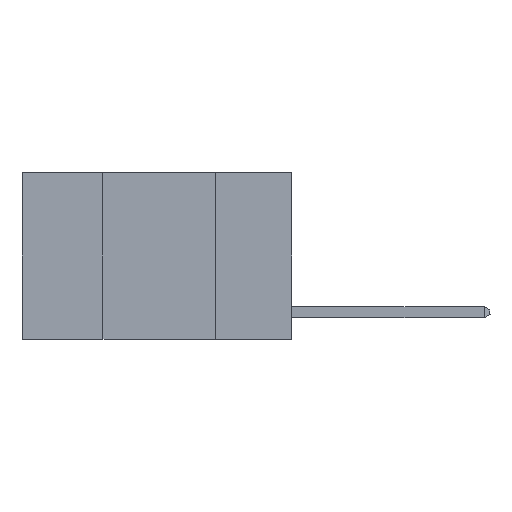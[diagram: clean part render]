
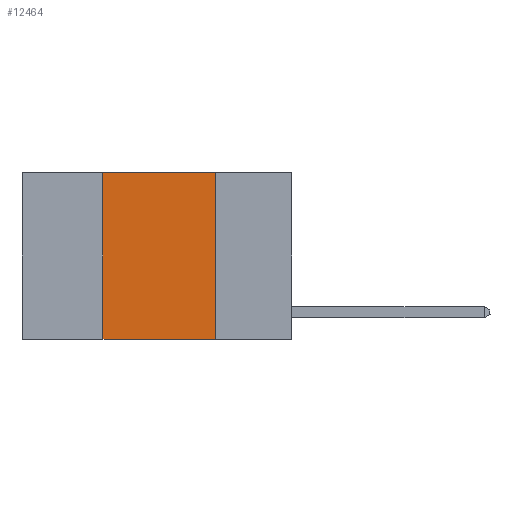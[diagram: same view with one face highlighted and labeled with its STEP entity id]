
A CAD part, left-side view. The second image highlights one B-rep face of the part: STEP entity #12464.
In plain terms, the highlighted planar face has unit normal (-1, 0, 0).
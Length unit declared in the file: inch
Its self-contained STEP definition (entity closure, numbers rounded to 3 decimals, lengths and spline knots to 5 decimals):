
#143 = LINE ( 'NONE', #9761, #8974 ) ;
#1460 = CARTESIAN_POINT ( 'NONE',  ( 0., 0.17, -0.37 ) ) ;
#2042 = VERTEX_POINT ( 'NONE', #4519 ) ;
#2284 = VECTOR ( 'NONE', #3607, 39.37008 ) ;
#2370 = EDGE_CURVE ( 'NONE', #4886, #2042, #3910, .T. ) ;
#2396 = LINE ( 'NONE', #17216, #2284 ) ;
#2710 = ORIENTED_EDGE ( 'NONE', *, *, #10743, .T. ) ;
#2777 = VERTEX_POINT ( 'NONE', #14789 ) ;
#3186 = ORIENTED_EDGE ( 'NONE', *, *, #12220, .F. ) ;
#3524 = LINE ( 'NONE', #13088, #8934 ) ;
#3607 = DIRECTION ( 'NONE',  ( 0., -1., 0. ) ) ;
#3910 = LINE ( 'NONE', #13058, #16837 ) ;
#4519 = CARTESIAN_POINT ( 'NONE',  ( 0., 0.42, 0. ) ) ;
#4886 = VERTEX_POINT ( 'NONE', #16364 ) ;
#5027 = ORIENTED_EDGE ( 'NONE', *, *, #2370, .F. ) ;
#5140 = PLANE ( 'NONE',  #10913 ) ;
#6248 = ORIENTED_EDGE ( 'NONE', *, *, #8086, .F. ) ;
#6345 = FACE_OUTER_BOUND ( 'NONE', #16952, .T. ) ;
#7720 = VERTEX_POINT ( 'NONE', #1460 ) ;
#7933 = CARTESIAN_POINT ( 'NONE',  ( 0., 0.6, 0. ) ) ;
#8086 = EDGE_CURVE ( 'NONE', #2042, #2777, #3524, .T. ) ;
#8934 = VECTOR ( 'NONE', #14060, 39.37008 ) ;
#8974 = VECTOR ( 'NONE', #16242, 39.37008 ) ;
#9211 = DIRECTION ( 'NONE',  ( 0., 0., 1. ) ) ;
#9761 = CARTESIAN_POINT ( 'NONE',  ( 0., 0.17, 0. ) ) ;
#10528 = DIRECTION ( 'NONE',  ( 0., 0., -1. ) ) ;
#10743 = EDGE_CURVE ( 'NONE', #4886, #7720, #2396, .T. ) ;
#10913 = AXIS2_PLACEMENT_3D ( 'NONE', #7933, #14294, #10528 ) ;
#12220 = EDGE_CURVE ( 'NONE', #2777, #7720, #143, .T. ) ;
#12464 = ADVANCED_FACE ( 'NONE', ( #6345 ), #5140, .F. ) ;
#13058 = CARTESIAN_POINT ( 'NONE',  ( 0., 0.42, 0. ) ) ;
#13088 = CARTESIAN_POINT ( 'NONE',  ( 0., 0.6, 0. ) ) ;
#14060 = DIRECTION ( 'NONE',  ( 0., -1., 0. ) ) ;
#14294 = DIRECTION ( 'NONE',  ( 1., 0., 0. ) ) ;
#14789 = CARTESIAN_POINT ( 'NONE',  ( 0., 0.17, 0. ) ) ;
#16242 = DIRECTION ( 'NONE',  ( 0., 0., -1. ) ) ;
#16364 = CARTESIAN_POINT ( 'NONE',  ( 0., 0.42, -0.37 ) ) ;
#16837 = VECTOR ( 'NONE', #9211, 39.37008 ) ;
#16952 = EDGE_LOOP ( 'NONE', ( #3186, #6248, #5027, #2710 ) ) ;
#17216 = CARTESIAN_POINT ( 'NONE',  ( 0., 0.6, -0.37 ) ) ;
